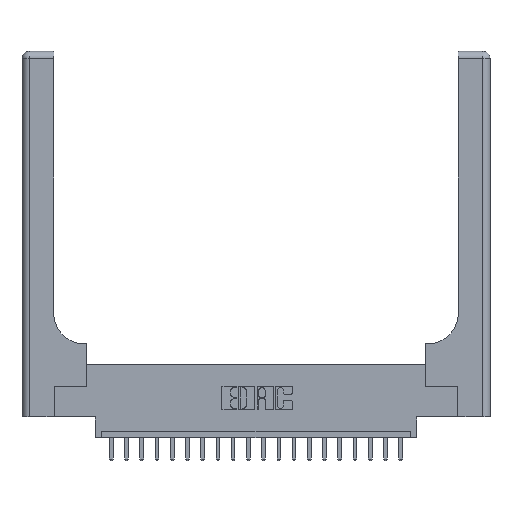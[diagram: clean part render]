
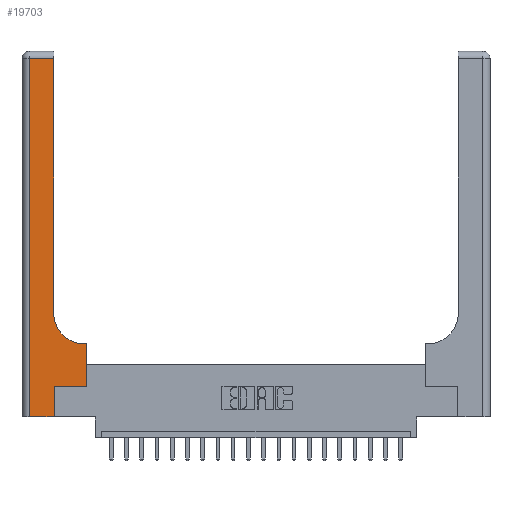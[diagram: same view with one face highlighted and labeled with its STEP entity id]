
A CAD part, top view. The second image highlights one B-rep face of the part: STEP entity #19703.
In plain terms, the highlighted planar face has unit normal (0, 0, 1).
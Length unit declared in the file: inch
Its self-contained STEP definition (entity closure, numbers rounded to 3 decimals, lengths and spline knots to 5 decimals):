
#228 = CARTESIAN_POINT ( 'NONE',  ( 0.51, 0.85, 0.37 ) ) ;
#403 = EDGE_LOOP ( 'NONE', ( #19320, #14930, #17578, #14576, #5932, #7334, #19606, #13988, #19751 ) ) ;
#416 = LINE ( 'NONE', #1608, #11212 ) ;
#788 = CIRCLE ( 'NONE', #9556, 0.25 ) ;
#1102 = DIRECTION ( 'NONE',  ( 1., 0., 0. ) ) ;
#1224 = CARTESIAN_POINT ( 'NONE',  ( 0.26, 0.85, 0.37 ) ) ;
#1457 = VECTOR ( 'NONE', #10525, 39.37008 ) ;
#1608 = CARTESIAN_POINT ( 'NONE',  ( 0.26, 0.6, 0.37 ) ) ;
#3281 = CARTESIAN_POINT ( 'NONE',  ( 0.528, 0.6, 0.37 ) ) ;
#3618 = AXIS2_PLACEMENT_3D ( 'NONE', #5331, #9410, #11589 ) ;
#3678 = LINE ( 'NONE', #10074, #9421 ) ;
#3842 = DIRECTION ( 'NONE',  ( 0., 0., -1. ) ) ;
#4065 = DIRECTION ( 'NONE',  ( 0., 1., 0. ) ) ;
#4239 = EDGE_CURVE ( 'NONE', #11249, #14553, #788, .T. ) ;
#4482 = CARTESIAN_POINT ( 'NONE',  ( 0.26, 2.94, 0.37 ) ) ;
#5184 = FACE_OUTER_BOUND ( 'NONE', #403, .T. ) ;
#5331 = CARTESIAN_POINT ( 'NONE',  ( 0., 3., 0.37 ) ) ;
#5599 = EDGE_CURVE ( 'NONE', #10337, #12254, #13859, .T. ) ;
#5932 = ORIENTED_EDGE ( 'NONE', *, *, #16839, .T. ) ;
#6818 = EDGE_CURVE ( 'NONE', #7089, #11249, #416, .T. ) ;
#6878 = DIRECTION ( 'NONE',  ( 0., 1., 0. ) ) ;
#7089 = VERTEX_POINT ( 'NONE', #3281 ) ;
#7280 = VERTEX_POINT ( 'NONE', #4482 ) ;
#7334 = ORIENTED_EDGE ( 'NONE', *, *, #20216, .T. ) ;
#7716 = DIRECTION ( 'NONE',  ( 1., 0., 0. ) ) ;
#8909 = CARTESIAN_POINT ( 'NONE',  ( 0.265, 0.25, 0.37 ) ) ;
#9410 = DIRECTION ( 'NONE',  ( 0., 0., -1. ) ) ;
#9421 = VECTOR ( 'NONE', #6878, 39.37008 ) ;
#9556 = AXIS2_PLACEMENT_3D ( 'NONE', #228, #3842, #15009 ) ;
#9966 = EDGE_CURVE ( 'NONE', #14553, #7280, #10849, .T. ) ;
#10074 = CARTESIAN_POINT ( 'NONE',  ( 0.265, 0., 0.37 ) ) ;
#10254 = PLANE ( 'NONE',  #3618 ) ;
#10337 = VERTEX_POINT ( 'NONE', #17479 ) ;
#10525 = DIRECTION ( 'NONE',  ( -1., 0., 0. ) ) ;
#10767 = VERTEX_POINT ( 'NONE', #17108 ) ;
#10849 = LINE ( 'NONE', #16206, #13181 ) ;
#10900 = VERTEX_POINT ( 'NONE', #16416 ) ;
#11212 = VECTOR ( 'NONE', #14598, 39.37008 ) ;
#11249 = VERTEX_POINT ( 'NONE', #15987 ) ;
#11589 = DIRECTION ( 'NONE',  ( -1., 0., 0. ) ) ;
#12019 = LINE ( 'NONE', #16791, #1457 ) ;
#12254 = VERTEX_POINT ( 'NONE', #17708 ) ;
#12419 = CARTESIAN_POINT ( 'NONE',  ( 0., 0., 0.37 ) ) ;
#12978 = EDGE_CURVE ( 'NONE', #7280, #13368, #12019, .T. ) ;
#13181 = VECTOR ( 'NONE', #16283, 39.37008 ) ;
#13198 = CARTESIAN_POINT ( 'NONE',  ( 0.528, 0.25, 0.37 ) ) ;
#13368 = VERTEX_POINT ( 'NONE', #17536 ) ;
#13859 = LINE ( 'NONE', #12419, #15096 ) ;
#13988 = ORIENTED_EDGE ( 'NONE', *, *, #6818, .T. ) ;
#14046 = DIRECTION ( 'NONE',  ( 0., -1., 0. ) ) ;
#14553 = VERTEX_POINT ( 'NONE', #1224 ) ;
#14576 = ORIENTED_EDGE ( 'NONE', *, *, #5599, .T. ) ;
#14598 = DIRECTION ( 'NONE',  ( -1., 0., 0. ) ) ;
#14774 = LINE ( 'NONE', #8909, #15257 ) ;
#14930 = ORIENTED_EDGE ( 'NONE', *, *, #12978, .T. ) ;
#15009 = DIRECTION ( 'NONE',  ( 1., 0., 0. ) ) ;
#15096 = VECTOR ( 'NONE', #7716, 39.37008 ) ;
#15219 = EDGE_CURVE ( 'NONE', #13368, #10337, #15495, .T. ) ;
#15257 = VECTOR ( 'NONE', #1102, 39.37008 ) ;
#15481 = EDGE_CURVE ( 'NONE', #10900, #7089, #16974, .T. ) ;
#15495 = LINE ( 'NONE', #20380, #20000 ) ;
#15987 = CARTESIAN_POINT ( 'NONE',  ( 0.51, 0.6, 0.37 ) ) ;
#16206 = CARTESIAN_POINT ( 'NONE',  ( 0.26, 3., 0.37 ) ) ;
#16283 = DIRECTION ( 'NONE',  ( 0., 1., 0. ) ) ;
#16416 = CARTESIAN_POINT ( 'NONE',  ( 0.528, 0.25, 0.37 ) ) ;
#16791 = CARTESIAN_POINT ( 'NONE',  ( 0., 2.94, 0.37 ) ) ;
#16839 = EDGE_CURVE ( 'NONE', #12254, #10767, #3678, .T. ) ;
#16974 = LINE ( 'NONE', #13198, #18489 ) ;
#17108 = CARTESIAN_POINT ( 'NONE',  ( 0.265, 0.25, 0.37 ) ) ;
#17479 = CARTESIAN_POINT ( 'NONE',  ( 0.06, 0., 0.37 ) ) ;
#17536 = CARTESIAN_POINT ( 'NONE',  ( 0.06, 2.94, 0.37 ) ) ;
#17578 = ORIENTED_EDGE ( 'NONE', *, *, #15219, .T. ) ;
#17708 = CARTESIAN_POINT ( 'NONE',  ( 0.265, 0., 0.37 ) ) ;
#18489 = VECTOR ( 'NONE', #4065, 39.37008 ) ;
#19320 = ORIENTED_EDGE ( 'NONE', *, *, #9966, .T. ) ;
#19606 = ORIENTED_EDGE ( 'NONE', *, *, #15481, .T. ) ;
#19703 = ADVANCED_FACE ( 'NONE', ( #5184 ), #10254, .F. ) ;
#19751 = ORIENTED_EDGE ( 'NONE', *, *, #4239, .T. ) ;
#20000 = VECTOR ( 'NONE', #14046, 39.37008 ) ;
#20216 = EDGE_CURVE ( 'NONE', #10767, #10900, #14774, .T. ) ;
#20380 = CARTESIAN_POINT ( 'NONE',  ( 0.06, 3., 0.37 ) ) ;
